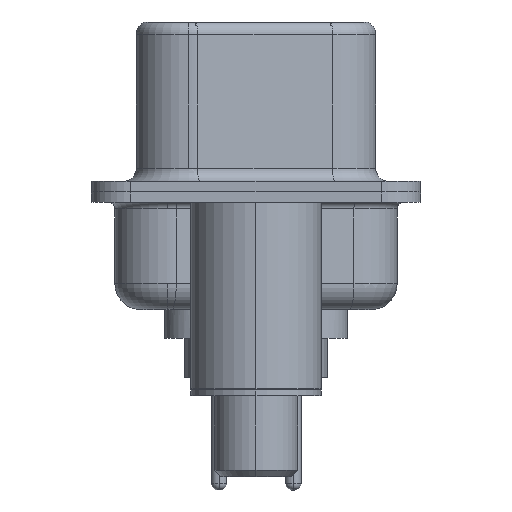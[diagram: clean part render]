
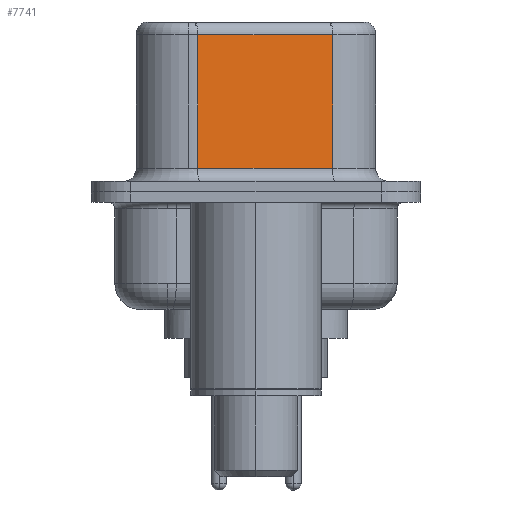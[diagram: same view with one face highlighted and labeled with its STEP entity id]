
A CAD part, left-side view. The second image highlights one B-rep face of the part: STEP entity #7741.
In plain terms, the highlighted planar face has unit normal (-0.985, -0.174, 0).
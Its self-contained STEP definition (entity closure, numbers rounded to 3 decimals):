
#589 = CARTESIAN_POINT ( 'NONE',  ( 4.58, -2.927, 0.9 ) ) ;
#982 = EDGE_CURVE ( 'NONE', #21983, #16371, #15288, .T. ) ;
#1220 = CARTESIAN_POINT ( 'NONE',  ( 3.67, 2.233, 0.9 ) ) ;
#1870 = DIRECTION ( 'NONE',  ( -0.174, 0.985, 0. ) ) ;
#2124 = VECTOR ( 'NONE', #7756, 1000. ) ;
#3282 = LINE ( 'NONE', #16898, #2124 ) ;
#3786 = DIRECTION ( 'NONE',  ( 0., 0., -1. ) ) ;
#3868 = VERTEX_POINT ( 'NONE', #15816 ) ;
#4245 = FACE_OUTER_BOUND ( 'NONE', #11658, .T. ) ;
#4706 = EDGE_CURVE ( 'NONE', #7576, #3868, #20118, .T. ) ;
#5632 = ORIENTED_EDGE ( 'NONE', *, *, #4706, .T. ) ;
#5661 = VECTOR ( 'NONE', #8783, 1000. ) ;
#5672 = VECTOR ( 'NONE', #1870, 1000. ) ;
#7576 = VERTEX_POINT ( 'NONE', #10450 ) ;
#7741 = ADVANCED_FACE ( 'NONE', ( #4245 ), #8686, .F. ) ;
#7756 = DIRECTION ( 'NONE',  ( 0., 0., -1. ) ) ;
#8589 = DIRECTION ( 'NONE',  ( -0.174, 0.985, 0. ) ) ;
#8636 = DIRECTION ( 'NONE',  ( 0.985, 0.174, 0. ) ) ;
#8667 = CARTESIAN_POINT ( 'NONE',  ( 4.58, -2.927, 6.52 ) ) ;
#8686 = PLANE ( 'NONE',  #16853 ) ;
#8783 = DIRECTION ( 'NONE',  ( 0.174, -0.985, 0. ) ) ;
#10450 = CARTESIAN_POINT ( 'NONE',  ( 4.58, -2.927, 6.02 ) ) ;
#10891 = CARTESIAN_POINT ( 'NONE',  ( 4.58, -2.927, 6.52 ) ) ;
#11658 = EDGE_LOOP ( 'NONE', ( #20569, #5632, #18658, #12835 ) ) ;
#12835 = ORIENTED_EDGE ( 'NONE', *, *, #982, .T. ) ;
#13676 = VECTOR ( 'NONE', #3786, 1000. ) ;
#15288 = LINE ( 'NONE', #20524, #5661 ) ;
#15816 = CARTESIAN_POINT ( 'NONE',  ( 3.67, 2.233, 6.02 ) ) ;
#16371 = VERTEX_POINT ( 'NONE', #589 ) ;
#16853 = AXIS2_PLACEMENT_3D ( 'NONE', #8667, #8636, #8589 ) ;
#16898 = CARTESIAN_POINT ( 'NONE',  ( 3.67, 2.233, 6.52 ) ) ;
#17048 = CARTESIAN_POINT ( 'NONE',  ( 4.58, -2.927, 6.02 ) ) ;
#18658 = ORIENTED_EDGE ( 'NONE', *, *, #20335, .T. ) ;
#19492 = EDGE_CURVE ( 'NONE', #7576, #16371, #23311, .T. ) ;
#20118 = LINE ( 'NONE', #17048, #5672 ) ;
#20335 = EDGE_CURVE ( 'NONE', #3868, #21983, #3282, .T. ) ;
#20524 = CARTESIAN_POINT ( 'NONE',  ( 4.58, -2.927, 0.9 ) ) ;
#20569 = ORIENTED_EDGE ( 'NONE', *, *, #19492, .F. ) ;
#21983 = VERTEX_POINT ( 'NONE', #1220 ) ;
#23311 = LINE ( 'NONE', #10891, #13676 ) ;
